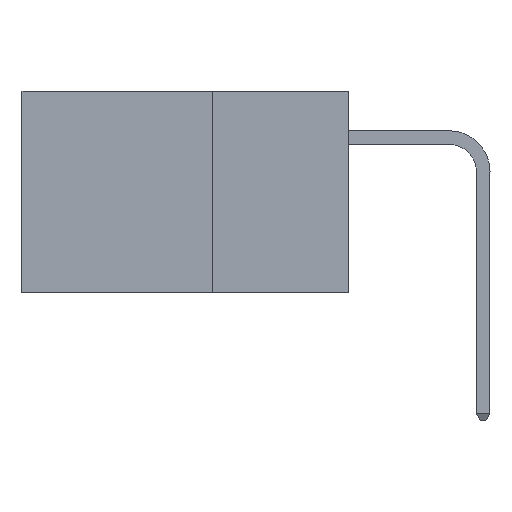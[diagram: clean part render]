
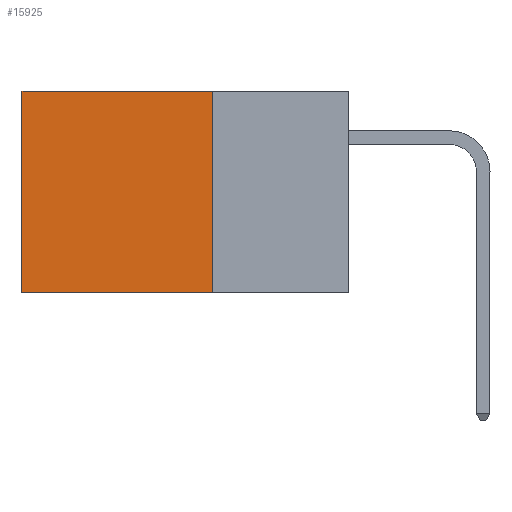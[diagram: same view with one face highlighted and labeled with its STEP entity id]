
A CAD part, left-side view. The second image highlights one B-rep face of the part: STEP entity #15925.
In plain terms, the highlighted planar face has unit normal (-1, 0, 0).
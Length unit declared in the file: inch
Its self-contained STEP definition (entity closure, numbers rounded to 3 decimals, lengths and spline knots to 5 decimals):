
#178 = EDGE_CURVE ( 'NONE', #23223, #26231, #11029, .T. ) ;
#1111 = CARTESIAN_POINT ( 'NONE',  ( 0.2875, 0.25, 0. ) ) ;
#1539 = EDGE_CURVE ( 'NONE', #4905, #26231, #27061, .T. ) ;
#2031 = VECTOR ( 'NONE', #23195, 39.37008 ) ;
#4711 = PLANE ( 'NONE',  #23959 ) ;
#4905 = VERTEX_POINT ( 'NONE', #23326 ) ;
#6865 = CARTESIAN_POINT ( 'NONE',  ( 0.2875, 0.25, 0. ) ) ;
#7095 = VECTOR ( 'NONE', #11173, 39.37008 ) ;
#8465 = CARTESIAN_POINT ( 'NONE',  ( 0.2875, 0.25, 0. ) ) ;
#8808 = EDGE_CURVE ( 'NONE', #22021, #4905, #23247, .T. ) ;
#8969 = DIRECTION ( 'NONE',  ( 1., 0., 0. ) ) ;
#9410 = EDGE_LOOP ( 'NONE', ( #22375, #12694, #25675, #17257 ) ) ;
#9771 = CARTESIAN_POINT ( 'NONE',  ( 0.2875, 0.25, -0.37 ) ) ;
#10174 = EDGE_CURVE ( 'NONE', #22021, #23223, #18229, .T. ) ;
#10295 = VECTOR ( 'NONE', #13937, 39.37008 ) ;
#10537 = DIRECTION ( 'NONE',  ( 0., 0., -1. ) ) ;
#11029 = LINE ( 'NONE', #12765, #15995 ) ;
#11173 = DIRECTION ( 'NONE',  ( 0., 0., -1. ) ) ;
#12694 = ORIENTED_EDGE ( 'NONE', *, *, #1539, .F. ) ;
#12765 = CARTESIAN_POINT ( 'NONE',  ( 0.2875, 0.6, 0. ) ) ;
#13888 = FACE_OUTER_BOUND ( 'NONE', #9410, .T. ) ;
#13937 = DIRECTION ( 'NONE',  ( 0., 1., 0. ) ) ;
#15925 = ADVANCED_FACE ( 'NONE', ( #13888 ), #4711, .F. ) ;
#15995 = VECTOR ( 'NONE', #10537, 39.37008 ) ;
#17257 = ORIENTED_EDGE ( 'NONE', *, *, #10174, .T. ) ;
#18229 = LINE ( 'NONE', #8465, #2031 ) ;
#20138 = CARTESIAN_POINT ( 'NONE',  ( 0.2875, 0.6, -0.37 ) ) ;
#21805 = CARTESIAN_POINT ( 'NONE',  ( 0.2875, 0.6, 0. ) ) ;
#22021 = VERTEX_POINT ( 'NONE', #1111 ) ;
#22375 = ORIENTED_EDGE ( 'NONE', *, *, #178, .T. ) ;
#23195 = DIRECTION ( 'NONE',  ( 0., 1., 0. ) ) ;
#23223 = VERTEX_POINT ( 'NONE', #21805 ) ;
#23247 = LINE ( 'NONE', #23751, #7095 ) ;
#23326 = CARTESIAN_POINT ( 'NONE',  ( 0.2875, 0.25, -0.37 ) ) ;
#23717 = DIRECTION ( 'NONE',  ( 0., 0., -1. ) ) ;
#23751 = CARTESIAN_POINT ( 'NONE',  ( 0.2875, 0.25, 0. ) ) ;
#23959 = AXIS2_PLACEMENT_3D ( 'NONE', #6865, #8969, #23717 ) ;
#25675 = ORIENTED_EDGE ( 'NONE', *, *, #8808, .F. ) ;
#26231 = VERTEX_POINT ( 'NONE', #20138 ) ;
#27061 = LINE ( 'NONE', #9771, #10295 ) ;
